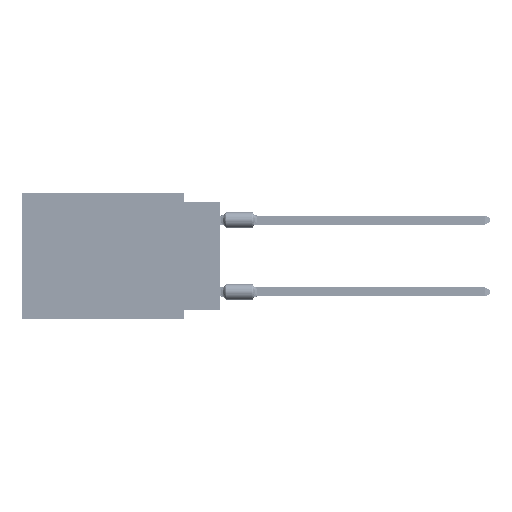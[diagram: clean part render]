
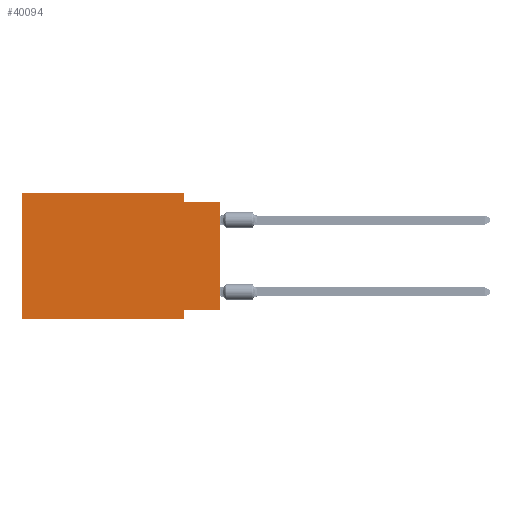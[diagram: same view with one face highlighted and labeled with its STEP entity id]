
A CAD part, left-side view. The second image highlights one B-rep face of the part: STEP entity #40094.
In plain terms, the highlighted planar face has unit normal (-1, 0, 0).
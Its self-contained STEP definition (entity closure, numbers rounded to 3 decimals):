
#2413 = LINE ( 'NONE', #28477, #3817 ) ;
#3072 = DIRECTION ( 'NONE',  ( 0., 0., 1. ) ) ;
#3457 = VERTEX_POINT ( 'NONE', #46246 ) ;
#3817 = VECTOR ( 'NONE', #3072, 1000. ) ;
#4567 = VECTOR ( 'NONE', #5638, 1000. ) ;
#5638 = DIRECTION ( 'NONE',  ( 0., 1., 0. ) ) ;
#6136 = CARTESIAN_POINT ( 'NONE',  ( 0., 2.54, -8.255 ) ) ;
#6675 = VECTOR ( 'NONE', #65996, 1000. ) ;
#7688 = CARTESIAN_POINT ( 'NONE',  ( 0., 13.97, 0. ) ) ;
#7701 = ORIENTED_EDGE ( 'NONE', *, *, #53066, .F. ) ;
#8689 = EDGE_CURVE ( 'NONE', #39868, #50607, #61222, .T. ) ;
#9429 = ORIENTED_EDGE ( 'NONE', *, *, #48091, .F. ) ;
#9686 = VECTOR ( 'NONE', #12653, 1000. ) ;
#12653 = DIRECTION ( 'NONE',  ( 0., -1., 0. ) ) ;
#12691 = PLANE ( 'NONE',  #62888 ) ;
#13351 = FACE_OUTER_BOUND ( 'NONE', #61547, .T. ) ;
#14073 = CARTESIAN_POINT ( 'NONE',  ( 0., 2.54, -8.89 ) ) ;
#14561 = DIRECTION ( 'NONE',  ( 0., -1., 0. ) ) ;
#14570 = LINE ( 'NONE', #35932, #6675 ) ;
#15677 = ORIENTED_EDGE ( 'NONE', *, *, #64580, .F. ) ;
#16722 = CARTESIAN_POINT ( 'NONE',  ( 0., 2.54, 0. ) ) ;
#17040 = VECTOR ( 'NONE', #51530, 1000. ) ;
#17658 = VERTEX_POINT ( 'NONE', #6136 ) ;
#20127 = CARTESIAN_POINT ( 'NONE',  ( 0., 0., -0.635 ) ) ;
#21835 = CARTESIAN_POINT ( 'NONE',  ( 0., 13.97, -8.89 ) ) ;
#25430 = LINE ( 'NONE', #31107, #59189 ) ;
#25752 = CARTESIAN_POINT ( 'NONE',  ( 0., 13.97, 0. ) ) ;
#27985 = ORIENTED_EDGE ( 'NONE', *, *, #57133, .T. ) ;
#28477 = CARTESIAN_POINT ( 'NONE',  ( 0., 13.97, 0. ) ) ;
#28581 = EDGE_CURVE ( 'NONE', #17658, #64686, #25430, .T. ) ;
#31107 = CARTESIAN_POINT ( 'NONE',  ( 0., 2.54, -8.89 ) ) ;
#31384 = EDGE_CURVE ( 'NONE', #57291, #39868, #54988, .T. ) ;
#33075 = DIRECTION ( 'NONE',  ( 0., 0., -1. ) ) ;
#33737 = DIRECTION ( 'NONE',  ( 1., 0., 0. ) ) ;
#35047 = CARTESIAN_POINT ( 'NONE',  ( 0., 2.54, -0.635 ) ) ;
#35470 = CARTESIAN_POINT ( 'NONE',  ( 0., 0., -8.255 ) ) ;
#35932 = CARTESIAN_POINT ( 'NONE',  ( 0., 0., 0. ) ) ;
#38565 = ORIENTED_EDGE ( 'NONE', *, *, #8689, .F. ) ;
#38816 = VECTOR ( 'NONE', #14561, 1000. ) ;
#39868 = VERTEX_POINT ( 'NONE', #16722 ) ;
#40094 = ADVANCED_FACE ( 'NONE', ( #13351 ), #12691, .F. ) ;
#40744 = ORIENTED_EDGE ( 'NONE', *, *, #28581, .F. ) ;
#42995 = EDGE_CURVE ( 'NONE', #55163, #3457, #14570, .T. ) ;
#46246 = CARTESIAN_POINT ( 'NONE',  ( 0., 0., -0.635 ) ) ;
#46280 = ORIENTED_EDGE ( 'NONE', *, *, #31384, .F. ) ;
#46805 = DIRECTION ( 'NONE',  ( 0., 0., -1. ) ) ;
#48081 = CARTESIAN_POINT ( 'NONE',  ( 0., 13.97, -8.89 ) ) ;
#48091 = EDGE_CURVE ( 'NONE', #55163, #17658, #56404, .T. ) ;
#50607 = VERTEX_POINT ( 'NONE', #35047 ) ;
#51391 = CARTESIAN_POINT ( 'NONE',  ( 0., 0., -8.255 ) ) ;
#51530 = DIRECTION ( 'NONE',  ( 0., 0., -1. ) ) ;
#51865 = CARTESIAN_POINT ( 'NONE',  ( 0., 2.54, 0. ) ) ;
#53066 = EDGE_CURVE ( 'NONE', #50607, #3457, #65892, .T. ) ;
#54988 = LINE ( 'NONE', #60644, #38816 ) ;
#55163 = VERTEX_POINT ( 'NONE', #35470 ) ;
#56404 = LINE ( 'NONE', #51391, #4567 ) ;
#57133 = EDGE_CURVE ( 'NONE', #65581, #64686, #57757, .T. ) ;
#57291 = VERTEX_POINT ( 'NONE', #25752 ) ;
#57757 = LINE ( 'NONE', #48081, #9686 ) ;
#59189 = VECTOR ( 'NONE', #46805, 1000. ) ;
#60644 = CARTESIAN_POINT ( 'NONE',  ( 0., 13.97, 0. ) ) ;
#61196 = DIRECTION ( 'NONE',  ( 0., -1., 0. ) ) ;
#61222 = LINE ( 'NONE', #51865, #17040 ) ;
#61547 = EDGE_LOOP ( 'NONE', ( #64991, #7701, #38565, #46280, #15677, #27985, #40744, #9429 ) ) ;
#62888 = AXIS2_PLACEMENT_3D ( 'NONE', #7688, #33737, #33075 ) ;
#64580 = EDGE_CURVE ( 'NONE', #65581, #57291, #2413, .T. ) ;
#64686 = VERTEX_POINT ( 'NONE', #14073 ) ;
#64991 = ORIENTED_EDGE ( 'NONE', *, *, #42995, .T. ) ;
#65581 = VERTEX_POINT ( 'NONE', #21835 ) ;
#65892 = LINE ( 'NONE', #20127, #66014 ) ;
#65996 = DIRECTION ( 'NONE',  ( 0., 0., 1. ) ) ;
#66014 = VECTOR ( 'NONE', #61196, 1000. ) ;
